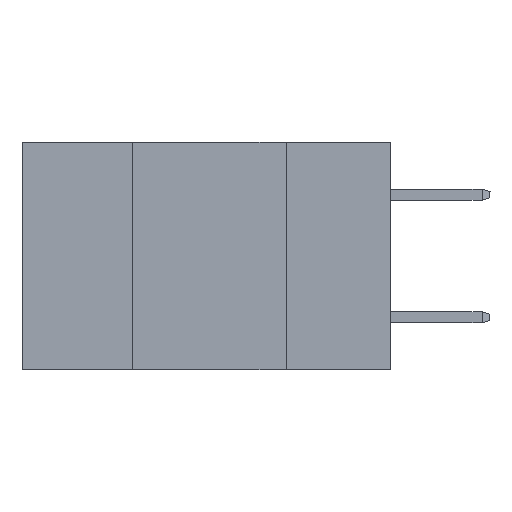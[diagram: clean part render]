
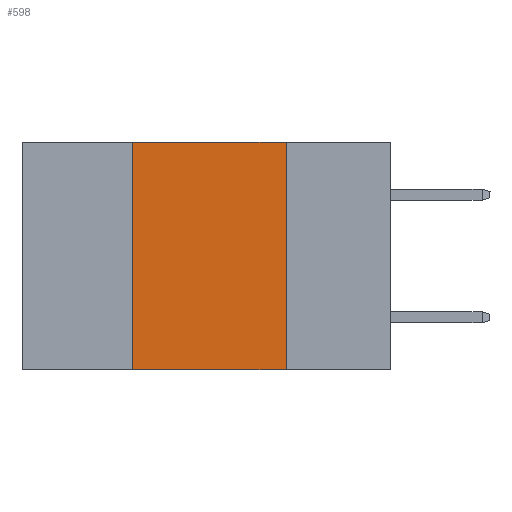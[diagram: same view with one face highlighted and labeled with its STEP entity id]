
A CAD part, left-side view. The second image highlights one B-rep face of the part: STEP entity #598.
In plain terms, the highlighted planar face has unit normal (-1, 0, 0).
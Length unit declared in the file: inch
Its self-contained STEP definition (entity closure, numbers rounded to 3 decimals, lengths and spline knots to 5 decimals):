
#77 = AXIS2_PLACEMENT_3D ( 'NONE', #13635, #7705, #524 ) ;
#524 = DIRECTION ( 'NONE',  ( 0., 0., -1. ) ) ;
#598 = ADVANCED_FACE ( 'NONE', ( #8762 ), #11538, .F. ) ;
#697 = LINE ( 'NONE', #3444, #13055 ) ;
#1322 = DIRECTION ( 'NONE',  ( 0., -1., 0. ) ) ;
#1926 = CARTESIAN_POINT ( 'NONE',  ( 0., 0.17, 0. ) ) ;
#2969 = ORIENTED_EDGE ( 'NONE', *, *, #7224, .F. ) ;
#3033 = VECTOR ( 'NONE', #6592, 39.37008 ) ;
#3444 = CARTESIAN_POINT ( 'NONE',  ( 0., 0.42, 0. ) ) ;
#3643 = VERTEX_POINT ( 'NONE', #4805 ) ;
#4143 = VECTOR ( 'NONE', #1322, 39.37008 ) ;
#4222 = EDGE_CURVE ( 'NONE', #5801, #3643, #10730, .T. ) ;
#4805 = CARTESIAN_POINT ( 'NONE',  ( 0., 0.17, -0.37 ) ) ;
#5765 = DIRECTION ( 'NONE',  ( 0., 0., -1. ) ) ;
#5801 = VERTEX_POINT ( 'NONE', #7027 ) ;
#5989 = EDGE_LOOP ( 'NONE', ( #2969, #10132, #9037, #13900 ) ) ;
#6304 = CARTESIAN_POINT ( 'NONE',  ( 0., 0.42, 0. ) ) ;
#6592 = DIRECTION ( 'NONE',  ( 0., -1., 0. ) ) ;
#6840 = EDGE_CURVE ( 'NONE', #5801, #6917, #697, .T. ) ;
#6917 = VERTEX_POINT ( 'NONE', #6304 ) ;
#7027 = CARTESIAN_POINT ( 'NONE',  ( 0., 0.42, -0.37 ) ) ;
#7064 = LINE ( 'NONE', #14992, #12480 ) ;
#7224 = EDGE_CURVE ( 'NONE', #13040, #3643, #7064, .T. ) ;
#7705 = DIRECTION ( 'NONE',  ( 1., 0., 0. ) ) ;
#8762 = FACE_OUTER_BOUND ( 'NONE', #5989, .T. ) ;
#9037 = ORIENTED_EDGE ( 'NONE', *, *, #6840, .F. ) ;
#10066 = EDGE_CURVE ( 'NONE', #6917, #13040, #10177, .T. ) ;
#10132 = ORIENTED_EDGE ( 'NONE', *, *, #10066, .F. ) ;
#10177 = LINE ( 'NONE', #13790, #3033 ) ;
#10679 = DIRECTION ( 'NONE',  ( 0., 0., 1. ) ) ;
#10730 = LINE ( 'NONE', #12963, #4143 ) ;
#11538 = PLANE ( 'NONE',  #77 ) ;
#12480 = VECTOR ( 'NONE', #5765, 39.37008 ) ;
#12963 = CARTESIAN_POINT ( 'NONE',  ( 0., 0.6, -0.37 ) ) ;
#13040 = VERTEX_POINT ( 'NONE', #1926 ) ;
#13055 = VECTOR ( 'NONE', #10679, 39.37008 ) ;
#13635 = CARTESIAN_POINT ( 'NONE',  ( 0., 0.6, 0. ) ) ;
#13790 = CARTESIAN_POINT ( 'NONE',  ( 0., 0.6, 0. ) ) ;
#13900 = ORIENTED_EDGE ( 'NONE', *, *, #4222, .T. ) ;
#14992 = CARTESIAN_POINT ( 'NONE',  ( 0., 0.17, 0. ) ) ;
